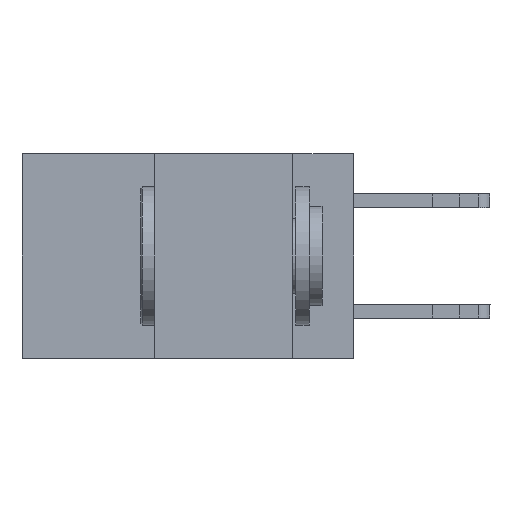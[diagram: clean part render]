
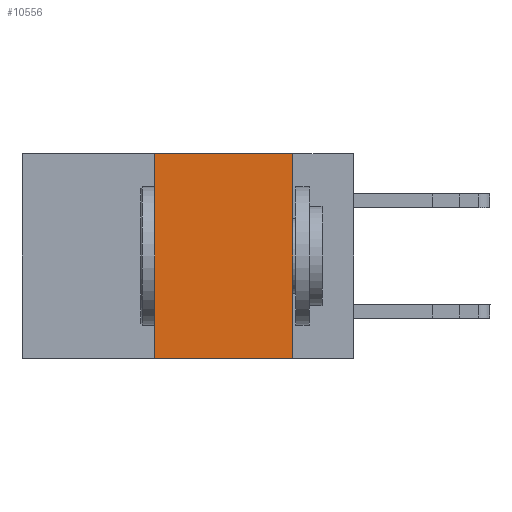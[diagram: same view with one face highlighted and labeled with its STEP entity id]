
A CAD part, left-side view. The second image highlights one B-rep face of the part: STEP entity #10556.
In plain terms, the highlighted planar face has unit normal (-1, 0, 0).
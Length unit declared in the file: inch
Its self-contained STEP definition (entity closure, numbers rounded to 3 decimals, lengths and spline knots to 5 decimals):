
#315 = LINE ( 'NONE', #11164, #6822 ) ;
#517 = EDGE_CURVE ( 'NONE', #5555, #1819, #17427, .T. ) ;
#736 = DIRECTION ( 'NONE',  ( 0., -1., 0. ) ) ;
#1819 = VERTEX_POINT ( 'NONE', #25392 ) ;
#5316 = VERTEX_POINT ( 'NONE', #14862 ) ;
#5417 = EDGE_CURVE ( 'NONE', #24896, #5316, #24021, .T. ) ;
#5555 = VERTEX_POINT ( 'NONE', #16148 ) ;
#6268 = DIRECTION ( 'NONE',  ( 1., 0., 0. ) ) ;
#6822 = VECTOR ( 'NONE', #736, 39.37008 ) ;
#7003 = CARTESIAN_POINT ( 'NONE',  ( 0., 0.36, 0. ) ) ;
#8436 = VECTOR ( 'NONE', #9356, 39.37008 ) ;
#8516 = CARTESIAN_POINT ( 'NONE',  ( 0., 0.6, 0. ) ) ;
#9356 = DIRECTION ( 'NONE',  ( 0., 0., -1. ) ) ;
#10139 = EDGE_CURVE ( 'NONE', #1819, #24896, #315, .T. ) ;
#10343 = FACE_OUTER_BOUND ( 'NONE', #18054, .T. ) ;
#10440 = EDGE_CURVE ( 'NONE', #5555, #5316, #18537, .T. ) ;
#10556 = ADVANCED_FACE ( 'NONE', ( #10343 ), #21626, .F. ) ;
#11164 = CARTESIAN_POINT ( 'NONE',  ( 0., 0.6, 0. ) ) ;
#11375 = ORIENTED_EDGE ( 'NONE', *, *, #10440, .T. ) ;
#12232 = ORIENTED_EDGE ( 'NONE', *, *, #517, .F. ) ;
#12309 = DIRECTION ( 'NONE',  ( 0., -1., 0. ) ) ;
#14862 = CARTESIAN_POINT ( 'NONE',  ( 0., 0.11, -0.37 ) ) ;
#15262 = ORIENTED_EDGE ( 'NONE', *, *, #5417, .F. ) ;
#15600 = DIRECTION ( 'NONE',  ( 0., 0., 1. ) ) ;
#15837 = CARTESIAN_POINT ( 'NONE',  ( 0., 0.11, 0. ) ) ;
#16148 = CARTESIAN_POINT ( 'NONE',  ( 0., 0.36, -0.37 ) ) ;
#17427 = LINE ( 'NONE', #7003, #24137 ) ;
#18054 = EDGE_LOOP ( 'NONE', ( #15262, #21365, #12232, #11375 ) ) ;
#18537 = LINE ( 'NONE', #27153, #23960 ) ;
#21073 = DIRECTION ( 'NONE',  ( 0., 0., -1. ) ) ;
#21365 = ORIENTED_EDGE ( 'NONE', *, *, #10139, .F. ) ;
#21626 = PLANE ( 'NONE',  #27109 ) ;
#23960 = VECTOR ( 'NONE', #12309, 39.37008 ) ;
#23974 = CARTESIAN_POINT ( 'NONE',  ( 0., 0.11, 0. ) ) ;
#24021 = LINE ( 'NONE', #15837, #8436 ) ;
#24137 = VECTOR ( 'NONE', #15600, 39.37008 ) ;
#24896 = VERTEX_POINT ( 'NONE', #23974 ) ;
#25392 = CARTESIAN_POINT ( 'NONE',  ( 0., 0.36, 0. ) ) ;
#27109 = AXIS2_PLACEMENT_3D ( 'NONE', #8516, #6268, #21073 ) ;
#27153 = CARTESIAN_POINT ( 'NONE',  ( 0., 0.6, -0.37 ) ) ;
